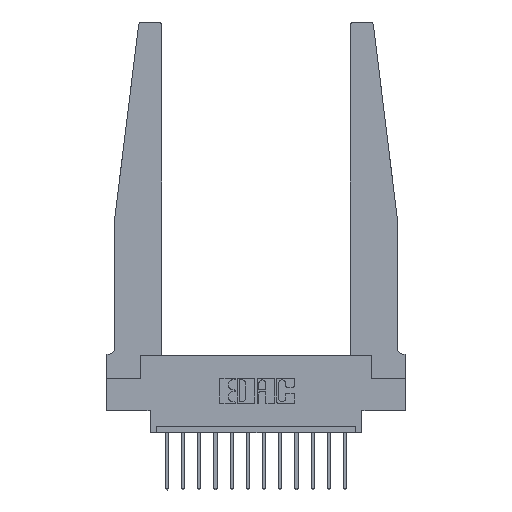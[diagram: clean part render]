
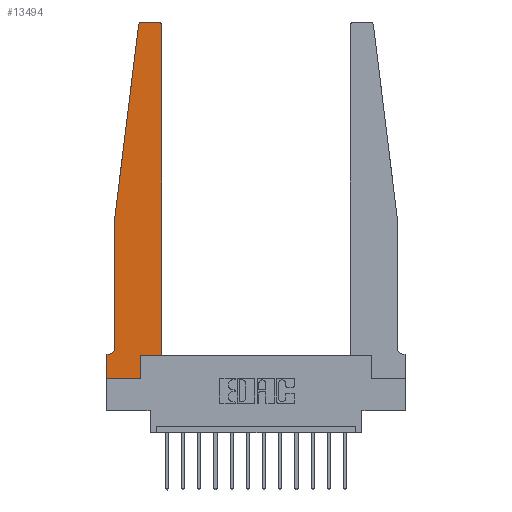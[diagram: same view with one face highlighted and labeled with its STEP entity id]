
A CAD part, top view. The second image highlights one B-rep face of the part: STEP entity #13494.
In plain terms, the highlighted planar face has unit normal (0, 0, 1).
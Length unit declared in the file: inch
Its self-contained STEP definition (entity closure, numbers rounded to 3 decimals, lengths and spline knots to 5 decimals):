
#117 = EDGE_CURVE ( 'NONE', #11422, #6530, #13764, .T. ) ;
#220 = VERTEX_POINT ( 'NONE', #5283 ) ;
#382 = CARTESIAN_POINT ( 'NONE',  ( 0., 0., 0.37 ) ) ;
#441 = CARTESIAN_POINT ( 'NONE',  ( 0.2605, 0.18, 0.37 ) ) ;
#726 = VECTOR ( 'NONE', #10595, 39.37008 ) ;
#899 = VECTOR ( 'NONE', #3439, 39.37008 ) ;
#1053 = DIRECTION ( 'NONE',  ( 0., 0., 1. ) ) ;
#1580 = ORIENTED_EDGE ( 'NONE', *, *, #10887, .T. ) ;
#1743 = CARTESIAN_POINT ( 'NONE',  ( 0., 0.1875, 0.37 ) ) ;
#1786 = LINE ( 'NONE', #15226, #6759 ) ;
#2147 = DIRECTION ( 'NONE',  ( 1., 0., 0. ) ) ;
#2198 = ORIENTED_EDGE ( 'NONE', *, *, #14717, .T. ) ;
#2444 = VECTOR ( 'NONE', #3619, 39.37008 ) ;
#2640 = DIRECTION ( 'NONE',  ( 0., 0., 1. ) ) ;
#3429 = EDGE_CURVE ( 'NONE', #220, #15259, #7997, .T. ) ;
#3439 = DIRECTION ( 'NONE',  ( 0., 1., 0. ) ) ;
#3619 = DIRECTION ( 'NONE',  ( 0., 1., 0. ) ) ;
#3780 = CARTESIAN_POINT ( 'NONE',  ( 0.065, 1.25, 0.37 ) ) ;
#3920 = CARTESIAN_POINT ( 'NONE',  ( 0.425, 2.72, 0.37 ) ) ;
#3983 = LINE ( 'NONE', #10333, #8201 ) ;
#4195 = ORIENTED_EDGE ( 'NONE', *, *, #9739, .T. ) ;
#4325 = VECTOR ( 'NONE', #13464, 39.37008 ) ;
#4571 = CARTESIAN_POINT ( 'NONE',  ( 0.425, 0.18, 0.37 ) ) ;
#4734 = VERTEX_POINT ( 'NONE', #1743 ) ;
#5033 = DIRECTION ( 'NONE',  ( 0., -1., 0. ) ) ;
#5093 = CARTESIAN_POINT ( 'NONE',  ( 0.395, 2.75, 0.37 ) ) ;
#5189 = ORIENTED_EDGE ( 'NONE', *, *, #13070, .T. ) ;
#5283 = CARTESIAN_POINT ( 'NONE',  ( 0.065, 0.2375, 0.37 ) ) ;
#5287 = VECTOR ( 'NONE', #9248, 39.37008 ) ;
#5347 = AXIS2_PLACEMENT_3D ( 'NONE', #7937, #2640, #7760 ) ;
#5554 = EDGE_CURVE ( 'NONE', #6530, #14758, #9683, .T. ) ;
#6429 = DIRECTION ( 'NONE',  ( -1., 0., 0. ) ) ;
#6436 = AXIS2_PLACEMENT_3D ( 'NONE', #10440, #10619, #9176 ) ;
#6464 = VERTEX_POINT ( 'NONE', #3920 ) ;
#6530 = VERTEX_POINT ( 'NONE', #441 ) ;
#6759 = VECTOR ( 'NONE', #6429, 39.37008 ) ;
#7097 = LINE ( 'NONE', #14473, #726 ) ;
#7223 = CARTESIAN_POINT ( 'NONE',  ( 0.2605, 0., 0.37 ) ) ;
#7302 = DIRECTION ( 'NONE',  ( 1., 0., 0. ) ) ;
#7760 = DIRECTION ( 'NONE',  ( 1., 0., 0. ) ) ;
#7832 = VERTEX_POINT ( 'NONE', #14653 ) ;
#7836 = CARTESIAN_POINT ( 'NONE',  ( 0.015, 0.1875, 0.37 ) ) ;
#7888 = VERTEX_POINT ( 'NONE', #5093 ) ;
#7937 = CARTESIAN_POINT ( 'NONE',  ( 0.27653, 2.72, 0.37 ) ) ;
#7979 = VECTOR ( 'NONE', #5033, 39.37008 ) ;
#7997 = CIRCLE ( 'NONE', #6436, 0.05 ) ;
#8116 = LINE ( 'NONE', #12996, #5287 ) ;
#8140 = PLANE ( 'NONE',  #15963 ) ;
#8201 = VECTOR ( 'NONE', #11664, 39.37008 ) ;
#8291 = EDGE_LOOP ( 'NONE', ( #12370, #5189, #15880, #12671, #15250, #1580, #4195, #8669, #13911, #14205, #12427, #2198 ) ) ;
#8550 = VERTEX_POINT ( 'NONE', #382 ) ;
#8669 = ORIENTED_EDGE ( 'NONE', *, *, #9275, .T. ) ;
#8758 = VERTEX_POINT ( 'NONE', #11512 ) ;
#8948 = EDGE_CURVE ( 'NONE', #7832, #9979, #8116, .T. ) ;
#9040 = LINE ( 'NONE', #12345, #899 ) ;
#9176 = DIRECTION ( 'NONE',  ( -1., 0., 0. ) ) ;
#9248 = DIRECTION ( 'NONE',  ( -0.122, -0.992, 0. ) ) ;
#9275 = EDGE_CURVE ( 'NONE', #8550, #11422, #3983, .T. ) ;
#9683 = LINE ( 'NONE', #4571, #4325 ) ;
#9739 = EDGE_CURVE ( 'NONE', #4734, #8550, #11734, .T. ) ;
#9742 = DIRECTION ( 'NONE',  ( 0., 0., 1. ) ) ;
#9979 = VERTEX_POINT ( 'NONE', #10122 ) ;
#10122 = CARTESIAN_POINT ( 'NONE',  ( 0.065, 1.25, 0.37 ) ) ;
#10333 = CARTESIAN_POINT ( 'NONE',  ( 0., 0., 0.37 ) ) ;
#10440 = CARTESIAN_POINT ( 'NONE',  ( 0.015, 0.2375, 0.37 ) ) ;
#10595 = DIRECTION ( 'NONE',  ( -1., 0., 0. ) ) ;
#10619 = DIRECTION ( 'NONE',  ( 0., 0., -1. ) ) ;
#10887 = EDGE_CURVE ( 'NONE', #15259, #4734, #1786, .T. ) ;
#11219 = CARTESIAN_POINT ( 'NONE',  ( 0.2605, 0.18, 0.37 ) ) ;
#11422 = VERTEX_POINT ( 'NONE', #7223 ) ;
#11512 = CARTESIAN_POINT ( 'NONE',  ( 0.27653, 2.75, 0.37 ) ) ;
#11664 = DIRECTION ( 'NONE',  ( 1., 0., 0. ) ) ;
#11734 = LINE ( 'NONE', #15174, #7979 ) ;
#12205 = FACE_OUTER_BOUND ( 'NONE', #8291, .T. ) ;
#12345 = CARTESIAN_POINT ( 'NONE',  ( 0.425, 0.18, 0.37 ) ) ;
#12353 = LINE ( 'NONE', #3780, #13569 ) ;
#12370 = ORIENTED_EDGE ( 'NONE', *, *, #13088, .T. ) ;
#12427 = ORIENTED_EDGE ( 'NONE', *, *, #13843, .T. ) ;
#12671 = ORIENTED_EDGE ( 'NONE', *, *, #14809, .T. ) ;
#12996 = CARTESIAN_POINT ( 'NONE',  ( 0.065, 1.25, 0.37 ) ) ;
#13070 = EDGE_CURVE ( 'NONE', #8758, #7832, #16177, .T. ) ;
#13088 = EDGE_CURVE ( 'NONE', #7888, #8758, #7097, .T. ) ;
#13176 = CIRCLE ( 'NONE', #13344, 0.03 ) ;
#13344 = AXIS2_PLACEMENT_3D ( 'NONE', #16233, #1053, #7302 ) ;
#13464 = DIRECTION ( 'NONE',  ( 1., 0., 0. ) ) ;
#13494 = ADVANCED_FACE ( 'NONE', ( #12205 ), #8140, .T. ) ;
#13569 = VECTOR ( 'NONE', #16393, 39.37008 ) ;
#13764 = LINE ( 'NONE', #11219, #2444 ) ;
#13843 = EDGE_CURVE ( 'NONE', #14758, #6464, #9040, .T. ) ;
#13911 = ORIENTED_EDGE ( 'NONE', *, *, #117, .T. ) ;
#14205 = ORIENTED_EDGE ( 'NONE', *, *, #5554, .T. ) ;
#14473 = CARTESIAN_POINT ( 'NONE',  ( 0.25, 2.75, 0.37 ) ) ;
#14653 = CARTESIAN_POINT ( 'NONE',  ( 0.24675, 2.72367, 0.37 ) ) ;
#14717 = EDGE_CURVE ( 'NONE', #6464, #7888, #13176, .T. ) ;
#14758 = VERTEX_POINT ( 'NONE', #14911 ) ;
#14809 = EDGE_CURVE ( 'NONE', #9979, #220, #12353, .T. ) ;
#14911 = CARTESIAN_POINT ( 'NONE',  ( 0.425, 0.18, 0.37 ) ) ;
#15174 = CARTESIAN_POINT ( 'NONE',  ( 0., 0., 0.37 ) ) ;
#15226 = CARTESIAN_POINT ( 'NONE',  ( 0.065, 0.1875, 0.37 ) ) ;
#15250 = ORIENTED_EDGE ( 'NONE', *, *, #3429, .T. ) ;
#15259 = VERTEX_POINT ( 'NONE', #7836 ) ;
#15880 = ORIENTED_EDGE ( 'NONE', *, *, #8948, .T. ) ;
#15963 = AXIS2_PLACEMENT_3D ( 'NONE', #16010, #9742, #2147 ) ;
#16010 = CARTESIAN_POINT ( 'NONE',  ( 0., 0.1875, 0.37 ) ) ;
#16177 = CIRCLE ( 'NONE', #5347, 0.03 ) ;
#16233 = CARTESIAN_POINT ( 'NONE',  ( 0.395, 2.72, 0.37 ) ) ;
#16393 = DIRECTION ( 'NONE',  ( 0., -1., 0. ) ) ;
